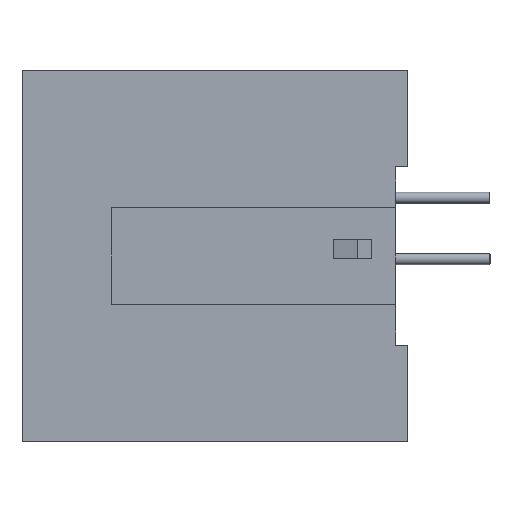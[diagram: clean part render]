
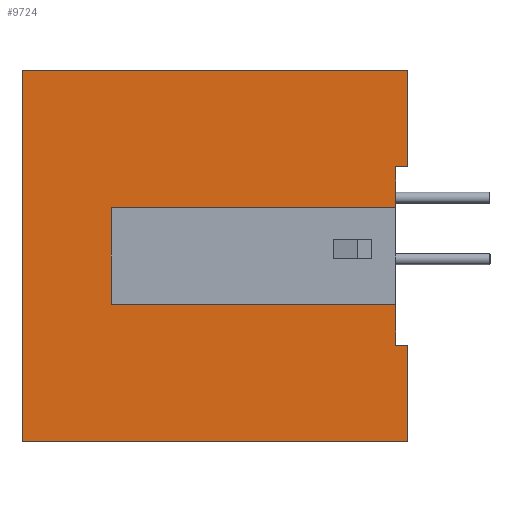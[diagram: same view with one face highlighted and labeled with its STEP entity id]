
A CAD part, left-side view. The second image highlights one B-rep face of the part: STEP entity #9724.
In plain terms, the highlighted planar face has unit normal (-1, 0, 0).
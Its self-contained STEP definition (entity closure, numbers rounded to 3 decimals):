
#114 = LINE ( 'NONE', #5069, #15453 ) ;
#339 = DIRECTION ( 'NONE',  ( 0., 1., 0. ) ) ;
#506 = ORIENTED_EDGE ( 'NONE', *, *, #9833, .F. ) ;
#741 = LINE ( 'NONE', #12592, #12904 ) ;
#841 = ORIENTED_EDGE ( 'NONE', *, *, #11135, .F. ) ;
#2098 = VECTOR ( 'NONE', #11508, 1000. ) ;
#2197 = DIRECTION ( 'NONE',  ( 0., 1., 0. ) ) ;
#2257 = LINE ( 'NONE', #5028, #13263 ) ;
#2270 = ORIENTED_EDGE ( 'NONE', *, *, #15441, .F. ) ;
#3048 = CARTESIAN_POINT ( 'NONE',  ( -27.5, -7.8, 0. ) ) ;
#3103 = LINE ( 'NONE', #13725, #4276 ) ;
#3462 = ORIENTED_EDGE ( 'NONE', *, *, #4807, .F. ) ;
#3626 = LINE ( 'NONE', #8745, #16252 ) ;
#4276 = VECTOR ( 'NONE', #10944, 1000. ) ;
#4422 = VERTEX_POINT ( 'NONE', #16260 ) ;
#4640 = CARTESIAN_POINT ( 'NONE',  ( -27.5, -0.3, 3.7 ) ) ;
#4807 = EDGE_CURVE ( 'NONE', #8317, #8480, #741, .T. ) ;
#5028 = CARTESIAN_POINT ( 'NONE',  ( -27.5, -0.3, -7.7 ) ) ;
#5058 = VERTEX_POINT ( 'NONE', #5167 ) ;
#5069 = CARTESIAN_POINT ( 'NONE',  ( -27.5, -7.8, 0. ) ) ;
#5167 = CARTESIAN_POINT ( 'NONE',  ( -27.5, -7.8, 3.7 ) ) ;
#5174 = CARTESIAN_POINT ( 'NONE',  ( -27.5, 7.7, -7.7 ) ) ;
#5233 = CARTESIAN_POINT ( 'NONE',  ( -27.5, -8.3, 3.7 ) ) ;
#5352 = AXIS2_PLACEMENT_3D ( 'NONE', #7829, #15589, #11714 ) ;
#5439 = VERTEX_POINT ( 'NONE', #5233 ) ;
#5618 = VECTOR ( 'NONE', #339, 1000. ) ;
#5746 = VERTEX_POINT ( 'NONE', #8492 ) ;
#6056 = LINE ( 'NONE', #13977, #6966 ) ;
#6214 = DIRECTION ( 'NONE',  ( 0., 1., 0. ) ) ;
#6755 = DIRECTION ( 'NONE',  ( 0., 0., -1. ) ) ;
#6764 = CARTESIAN_POINT ( 'NONE',  ( -27.5, 4., -1.8 ) ) ;
#6929 = CARTESIAN_POINT ( 'NONE',  ( -27.5, 4., 1.8 ) ) ;
#6966 = VECTOR ( 'NONE', #13893, 1000. ) ;
#7002 = LINE ( 'NONE', #3048, #8298 ) ;
#7042 = EDGE_CURVE ( 'NONE', #14660, #4422, #3626, .T. ) ;
#7058 = CARTESIAN_POINT ( 'NONE',  ( -27.5, -0.3, 1.8 ) ) ;
#7470 = LINE ( 'NONE', #15393, #9761 ) ;
#7539 = LINE ( 'NONE', #12685, #2098 ) ;
#7599 = VERTEX_POINT ( 'NONE', #9730 ) ;
#7793 = ORIENTED_EDGE ( 'NONE', *, *, #15893, .F. ) ;
#7829 = CARTESIAN_POINT ( 'NONE',  ( -27.5, -8.62, -8.008 ) ) ;
#7912 = ORIENTED_EDGE ( 'NONE', *, *, #15794, .F. ) ;
#7956 = ORIENTED_EDGE ( 'NONE', *, *, #8062, .F. ) ;
#8062 = EDGE_CURVE ( 'NONE', #5058, #7599, #114, .T. ) ;
#8073 = PLANE ( 'NONE',  #5352 ) ;
#8298 = VECTOR ( 'NONE', #6755, 1000. ) ;
#8317 = VERTEX_POINT ( 'NONE', #13657 ) ;
#8480 = VERTEX_POINT ( 'NONE', #11934 ) ;
#8492 = CARTESIAN_POINT ( 'NONE',  ( -27.5, -7.8, -1.8 ) ) ;
#8627 = CARTESIAN_POINT ( 'NONE',  ( -27.5, -7.8, -3.7 ) ) ;
#8745 = CARTESIAN_POINT ( 'NONE',  ( -27.5, 7.7, 0. ) ) ;
#8866 = EDGE_CURVE ( 'NONE', #13948, #5746, #7539, .T. ) ;
#8923 = VERTEX_POINT ( 'NONE', #6929 ) ;
#9622 = EDGE_CURVE ( 'NONE', #12293, #4422, #12035, .T. ) ;
#9724 = ADVANCED_FACE ( 'NONE', ( #14651 ), #8073, .F. ) ;
#9730 = CARTESIAN_POINT ( 'NONE',  ( -27.5, -7.8, 1.8 ) ) ;
#9761 = VECTOR ( 'NONE', #11441, 1000. ) ;
#9833 = EDGE_CURVE ( 'NONE', #13926, #8317, #3103, .T. ) ;
#9937 = EDGE_LOOP ( 'NONE', ( #841, #10911, #14995, #11432, #3462, #506, #15594, #14654, #7793, #7912, #7956, #2270 ) ) ;
#10427 = EDGE_CURVE ( 'NONE', #5746, #13926, #7002, .T. ) ;
#10911 = ORIENTED_EDGE ( 'NONE', *, *, #9622, .T. ) ;
#10944 = DIRECTION ( 'NONE',  ( 0., -1., 0. ) ) ;
#11135 = EDGE_CURVE ( 'NONE', #12293, #5439, #6056, .T. ) ;
#11379 = DIRECTION ( 'NONE',  ( 0., 0., 1. ) ) ;
#11432 = ORIENTED_EDGE ( 'NONE', *, *, #15957, .F. ) ;
#11441 = DIRECTION ( 'NONE',  ( 0., 0., -1. ) ) ;
#11508 = DIRECTION ( 'NONE',  ( 0., -1., 0. ) ) ;
#11714 = DIRECTION ( 'NONE',  ( 0., 1., 0. ) ) ;
#11790 = LINE ( 'NONE', #7058, #12185 ) ;
#11934 = CARTESIAN_POINT ( 'NONE',  ( -27.5, -8.3, -7.7 ) ) ;
#12035 = LINE ( 'NONE', #14409, #5618 ) ;
#12185 = VECTOR ( 'NONE', #13552, 1000. ) ;
#12293 = VERTEX_POINT ( 'NONE', #14475 ) ;
#12592 = CARTESIAN_POINT ( 'NONE',  ( -27.5, -8.3, 0. ) ) ;
#12685 = CARTESIAN_POINT ( 'NONE',  ( -27.5, -0.3, -1.8 ) ) ;
#12904 = VECTOR ( 'NONE', #16464, 1000. ) ;
#13263 = VECTOR ( 'NONE', #6214, 1000. ) ;
#13487 = LINE ( 'NONE', #4640, #16480 ) ;
#13552 = DIRECTION ( 'NONE',  ( 0., 1., 0. ) ) ;
#13657 = CARTESIAN_POINT ( 'NONE',  ( -27.5, -8.3, -3.7 ) ) ;
#13725 = CARTESIAN_POINT ( 'NONE',  ( -27.5, -0.3, -3.7 ) ) ;
#13893 = DIRECTION ( 'NONE',  ( 0., 0., -1. ) ) ;
#13926 = VERTEX_POINT ( 'NONE', #8627 ) ;
#13948 = VERTEX_POINT ( 'NONE', #6764 ) ;
#13977 = CARTESIAN_POINT ( 'NONE',  ( -27.5, -8.3, 0. ) ) ;
#14409 = CARTESIAN_POINT ( 'NONE',  ( -27.5, -0.3, 7.7 ) ) ;
#14475 = CARTESIAN_POINT ( 'NONE',  ( -27.5, -8.3, 7.7 ) ) ;
#14651 = FACE_OUTER_BOUND ( 'NONE', #9937, .T. ) ;
#14654 = ORIENTED_EDGE ( 'NONE', *, *, #8866, .F. ) ;
#14660 = VERTEX_POINT ( 'NONE', #5174 ) ;
#14995 = ORIENTED_EDGE ( 'NONE', *, *, #7042, .F. ) ;
#15393 = CARTESIAN_POINT ( 'NONE',  ( -27.5, 4., 0. ) ) ;
#15441 = EDGE_CURVE ( 'NONE', #5439, #5058, #13487, .T. ) ;
#15453 = VECTOR ( 'NONE', #15518, 1000. ) ;
#15518 = DIRECTION ( 'NONE',  ( 0., 0., -1. ) ) ;
#15589 = DIRECTION ( 'NONE',  ( 1., 0., 0. ) ) ;
#15594 = ORIENTED_EDGE ( 'NONE', *, *, #10427, .F. ) ;
#15794 = EDGE_CURVE ( 'NONE', #7599, #8923, #11790, .T. ) ;
#15893 = EDGE_CURVE ( 'NONE', #8923, #13948, #7470, .T. ) ;
#15957 = EDGE_CURVE ( 'NONE', #8480, #14660, #2257, .T. ) ;
#16252 = VECTOR ( 'NONE', #11379, 1000. ) ;
#16260 = CARTESIAN_POINT ( 'NONE',  ( -27.5, 7.7, 7.7 ) ) ;
#16464 = DIRECTION ( 'NONE',  ( 0., 0., -1. ) ) ;
#16480 = VECTOR ( 'NONE', #2197, 1000. ) ;
